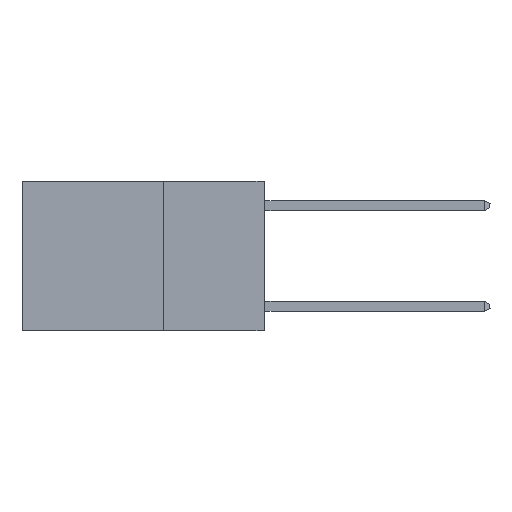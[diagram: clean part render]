
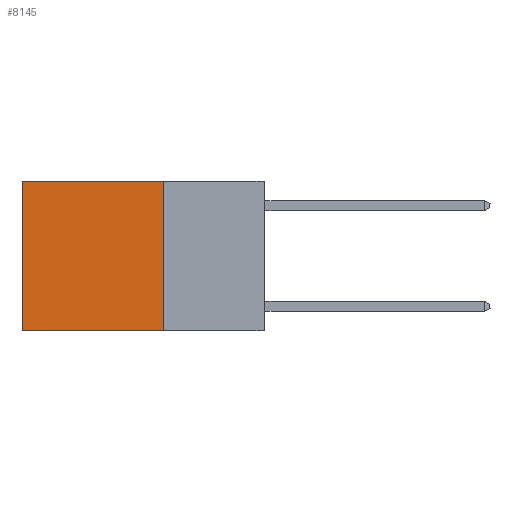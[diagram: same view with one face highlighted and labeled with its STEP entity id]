
A CAD part, left-side view. The second image highlights one B-rep face of the part: STEP entity #8145.
In plain terms, the highlighted planar face has unit normal (-1, 0, 0).
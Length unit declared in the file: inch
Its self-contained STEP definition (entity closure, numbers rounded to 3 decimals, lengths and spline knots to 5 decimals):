
#16 = DIRECTION ( 'NONE',  ( 0., 0., -1. ) ) ;
#108 = DIRECTION ( 'NONE',  ( 0., 0., -1. ) ) ;
#1121 = CARTESIAN_POINT ( 'NONE',  ( 0.2625, 0.25, -0.37 ) ) ;
#1787 = CARTESIAN_POINT ( 'NONE',  ( 0.2625, 0.6, 0. ) ) ;
#2409 = EDGE_CURVE ( 'NONE', #11551, #6973, #6421, .T. ) ;
#3103 = EDGE_LOOP ( 'NONE', ( #11491, #15460, #6867, #15705 ) ) ;
#4240 = VECTOR ( 'NONE', #5566, 39.37008 ) ;
#4961 = VECTOR ( 'NONE', #5301, 39.37008 ) ;
#5208 = LINE ( 'NONE', #14966, #4961 ) ;
#5301 = DIRECTION ( 'NONE',  ( 0., 1., 0. ) ) ;
#5566 = DIRECTION ( 'NONE',  ( 0., 0., -1. ) ) ;
#6421 = LINE ( 'NONE', #7620, #14400 ) ;
#6867 = ORIENTED_EDGE ( 'NONE', *, *, #14153, .F. ) ;
#6973 = VERTEX_POINT ( 'NONE', #1787 ) ;
#7620 = CARTESIAN_POINT ( 'NONE',  ( 0.2625, 0.25, 0. ) ) ;
#7889 = LINE ( 'NONE', #15472, #4240 ) ;
#8145 = ADVANCED_FACE ( 'NONE', ( #13745 ), #15129, .F. ) ;
#8575 = CARTESIAN_POINT ( 'NONE',  ( 0.2625, 0.25, 0. ) ) ;
#9567 = CARTESIAN_POINT ( 'NONE',  ( 0.2625, 0.6, -0.37 ) ) ;
#10248 = VERTEX_POINT ( 'NONE', #9567 ) ;
#10679 = VERTEX_POINT ( 'NONE', #1121 ) ;
#11168 = CARTESIAN_POINT ( 'NONE',  ( 0.2625, 0.6, 0. ) ) ;
#11491 = ORIENTED_EDGE ( 'NONE', *, *, #13151, .T. ) ;
#11551 = VERTEX_POINT ( 'NONE', #13567 ) ;
#12162 = AXIS2_PLACEMENT_3D ( 'NONE', #8575, #12308, #16 ) ;
#12308 = DIRECTION ( 'NONE',  ( 1., 0., 0. ) ) ;
#12663 = EDGE_CURVE ( 'NONE', #10679, #10248, #5208, .T. ) ;
#13151 = EDGE_CURVE ( 'NONE', #6973, #10248, #14956, .T. ) ;
#13502 = DIRECTION ( 'NONE',  ( 0., 1., 0. ) ) ;
#13567 = CARTESIAN_POINT ( 'NONE',  ( 0.2625, 0.25, 0. ) ) ;
#13745 = FACE_OUTER_BOUND ( 'NONE', #3103, .T. ) ;
#14153 = EDGE_CURVE ( 'NONE', #11551, #10679, #7889, .T. ) ;
#14400 = VECTOR ( 'NONE', #13502, 39.37008 ) ;
#14522 = VECTOR ( 'NONE', #108, 39.37008 ) ;
#14956 = LINE ( 'NONE', #11168, #14522 ) ;
#14966 = CARTESIAN_POINT ( 'NONE',  ( 0.2625, 0.25, -0.37 ) ) ;
#15129 = PLANE ( 'NONE',  #12162 ) ;
#15460 = ORIENTED_EDGE ( 'NONE', *, *, #12663, .F. ) ;
#15472 = CARTESIAN_POINT ( 'NONE',  ( 0.2625, 0.25, 0. ) ) ;
#15705 = ORIENTED_EDGE ( 'NONE', *, *, #2409, .T. ) ;
